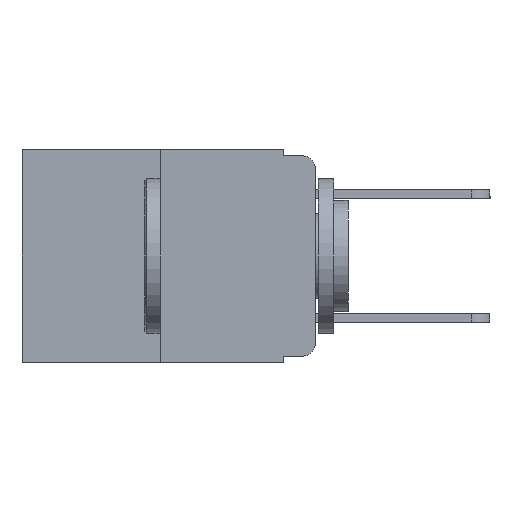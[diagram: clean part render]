
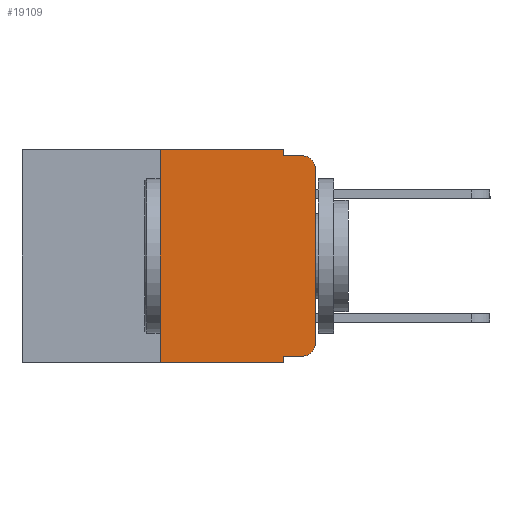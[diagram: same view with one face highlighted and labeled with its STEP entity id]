
A CAD part, left-side view. The second image highlights one B-rep face of the part: STEP entity #19109.
In plain terms, the highlighted planar face has unit normal (-1, 0, 0).
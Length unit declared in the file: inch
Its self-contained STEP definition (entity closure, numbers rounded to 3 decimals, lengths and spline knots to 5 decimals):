
#357 = PLANE ( 'NONE',  #17387 ) ;
#486 = CARTESIAN_POINT ( 'NONE',  ( 0., 0.25, -0.343 ) ) ;
#585 = ORIENTED_EDGE ( 'NONE', *, *, #21473, .F. ) ;
#590 = DIRECTION ( 'NONE',  ( 0., -1., 0. ) ) ;
#603 = EDGE_CURVE ( 'NONE', #18510, #14778, #22321, .T. ) ;
#617 = VECTOR ( 'NONE', #19484, 39.37008 ) ;
#928 = EDGE_CURVE ( 'NONE', #18746, #7361, #19233, .T. ) ;
#955 = CARTESIAN_POINT ( 'NONE',  ( 0., 0.25, 0. ) ) ;
#1152 = EDGE_CURVE ( 'NONE', #2774, #6932, #14683, .T. ) ;
#1568 = CARTESIAN_POINT ( 'NONE',  ( 0., 0.02, -0.03 ) ) ;
#2133 = DIRECTION ( 'NONE',  ( 0., 0., -1. ) ) ;
#2232 = DIRECTION ( 'NONE',  ( 1., 0., 0. ) ) ;
#2328 = CARTESIAN_POINT ( 'NONE',  ( 0., 0.473, 0. ) ) ;
#2392 = CARTESIAN_POINT ( 'NONE',  ( 0., 0.02, -0.313 ) ) ;
#2570 = CARTESIAN_POINT ( 'NONE',  ( 0., 0.051, 0. ) ) ;
#2749 = DIRECTION ( 'NONE',  ( 0., 0., 1. ) ) ;
#2774 = VERTEX_POINT ( 'NONE', #21116 ) ;
#2879 = ORIENTED_EDGE ( 'NONE', *, *, #20660, .F. ) ;
#3184 = CARTESIAN_POINT ( 'NONE',  ( 0., 0.051, -0.01 ) ) ;
#3417 = DIRECTION ( 'NONE',  ( 0., 0., -1. ) ) ;
#3971 = CARTESIAN_POINT ( 'NONE',  ( 0., 0.051, 0. ) ) ;
#4167 = DIRECTION ( 'NONE',  ( 0., -1., 0. ) ) ;
#4232 = DIRECTION ( 'NONE',  ( 0., 0., -1. ) ) ;
#4246 = VERTEX_POINT ( 'NONE', #9905 ) ;
#4282 = ORIENTED_EDGE ( 'NONE', *, *, #23324, .F. ) ;
#4376 = CARTESIAN_POINT ( 'NONE',  ( 0., 0., 0. ) ) ;
#4952 = LINE ( 'NONE', #2570, #9179 ) ;
#5584 = EDGE_CURVE ( 'NONE', #6932, #18746, #22696, .T. ) ;
#6523 = CARTESIAN_POINT ( 'NONE',  ( 0., 0., -0.313 ) ) ;
#6932 = VERTEX_POINT ( 'NONE', #18890 ) ;
#7202 = LINE ( 'NONE', #3971, #16274 ) ;
#7361 = VERTEX_POINT ( 'NONE', #16422 ) ;
#7391 = ORIENTED_EDGE ( 'NONE', *, *, #12608, .T. ) ;
#7814 = AXIS2_PLACEMENT_3D ( 'NONE', #2392, #15057, #4232 ) ;
#9116 = AXIS2_PLACEMENT_3D ( 'NONE', #1568, #14210, #3417 ) ;
#9179 = VECTOR ( 'NONE', #20684, 39.37008 ) ;
#9612 = CARTESIAN_POINT ( 'NONE',  ( 0., 0.051, -0.333 ) ) ;
#9837 = VECTOR ( 'NONE', #590, 39.37008 ) ;
#9905 = CARTESIAN_POINT ( 'NONE',  ( 0., 0.051, 0. ) ) ;
#10243 = LINE ( 'NONE', #3184, #617 ) ;
#10471 = LINE ( 'NONE', #2328, #15323 ) ;
#10510 = CARTESIAN_POINT ( 'NONE',  ( 0., 0.051, -0.01 ) ) ;
#10976 = DIRECTION ( 'NONE',  ( 0., -1., 0. ) ) ;
#11745 = EDGE_CURVE ( 'NONE', #18510, #19465, #19569, .T. ) ;
#11791 = FACE_OUTER_BOUND ( 'NONE', #19582, .T. ) ;
#11908 = ORIENTED_EDGE ( 'NONE', *, *, #22295, .F. ) ;
#12148 = VECTOR ( 'NONE', #10976, 39.37008 ) ;
#12307 = CARTESIAN_POINT ( 'NONE',  ( 0., 0.02, -0.01 ) ) ;
#12441 = CARTESIAN_POINT ( 'NONE',  ( 0., 0.473, -0.343 ) ) ;
#12608 = EDGE_CURVE ( 'NONE', #7361, #14802, #15258, .T. ) ;
#13023 = CARTESIAN_POINT ( 'NONE',  ( 0., 0.473, 0. ) ) ;
#14079 = ORIENTED_EDGE ( 'NONE', *, *, #5584, .T. ) ;
#14210 = DIRECTION ( 'NONE',  ( -1., 0., 0. ) ) ;
#14397 = VECTOR ( 'NONE', #2749, 39.37008 ) ;
#14683 = LINE ( 'NONE', #9612, #9837 ) ;
#14732 = VECTOR ( 'NONE', #20828, 39.37008 ) ;
#14778 = VERTEX_POINT ( 'NONE', #19548 ) ;
#14802 = VERTEX_POINT ( 'NONE', #12307 ) ;
#14880 = DIRECTION ( 'NONE',  ( 0., 0., -1. ) ) ;
#15057 = DIRECTION ( 'NONE',  ( -1., 0., 0. ) ) ;
#15258 = CIRCLE ( 'NONE', #9116, 0.02 ) ;
#15323 = VECTOR ( 'NONE', #4167, 39.37008 ) ;
#15599 = ORIENTED_EDGE ( 'NONE', *, *, #11745, .F. ) ;
#16274 = VECTOR ( 'NONE', #2133, 39.37008 ) ;
#16422 = CARTESIAN_POINT ( 'NONE',  ( 0., 0., -0.03 ) ) ;
#17387 = AXIS2_PLACEMENT_3D ( 'NONE', #13023, #2232, #14880 ) ;
#17894 = ORIENTED_EDGE ( 'NONE', *, *, #603, .T. ) ;
#18510 = VERTEX_POINT ( 'NONE', #486 ) ;
#18746 = VERTEX_POINT ( 'NONE', #6523 ) ;
#18857 = VERTEX_POINT ( 'NONE', #10510 ) ;
#18890 = CARTESIAN_POINT ( 'NONE',  ( 0., 0.02, -0.333 ) ) ;
#19109 = ADVANCED_FACE ( 'NONE', ( #11791 ), #357, .F. ) ;
#19233 = LINE ( 'NONE', #4376, #14397 ) ;
#19465 = VERTEX_POINT ( 'NONE', #21271 ) ;
#19484 = DIRECTION ( 'NONE',  ( 0., -1., 0. ) ) ;
#19548 = CARTESIAN_POINT ( 'NONE',  ( 0., 0.051, -0.343 ) ) ;
#19569 = LINE ( 'NONE', #955, #14732 ) ;
#19582 = EDGE_LOOP ( 'NONE', ( #22637, #7391, #11908, #2879, #4282, #15599, #17894, #585, #21248, #14079 ) ) ;
#20660 = EDGE_CURVE ( 'NONE', #4246, #18857, #7202, .T. ) ;
#20684 = DIRECTION ( 'NONE',  ( 0., 0., -1. ) ) ;
#20828 = DIRECTION ( 'NONE',  ( 0., 0., 1. ) ) ;
#21116 = CARTESIAN_POINT ( 'NONE',  ( 0., 0.051, -0.333 ) ) ;
#21248 = ORIENTED_EDGE ( 'NONE', *, *, #1152, .T. ) ;
#21271 = CARTESIAN_POINT ( 'NONE',  ( 0., 0.25, 0. ) ) ;
#21473 = EDGE_CURVE ( 'NONE', #2774, #14778, #4952, .T. ) ;
#22295 = EDGE_CURVE ( 'NONE', #18857, #14802, #10243, .T. ) ;
#22321 = LINE ( 'NONE', #12441, #12148 ) ;
#22637 = ORIENTED_EDGE ( 'NONE', *, *, #928, .T. ) ;
#22696 = CIRCLE ( 'NONE', #7814, 0.02 ) ;
#23324 = EDGE_CURVE ( 'NONE', #19465, #4246, #10471, .T. ) ;
